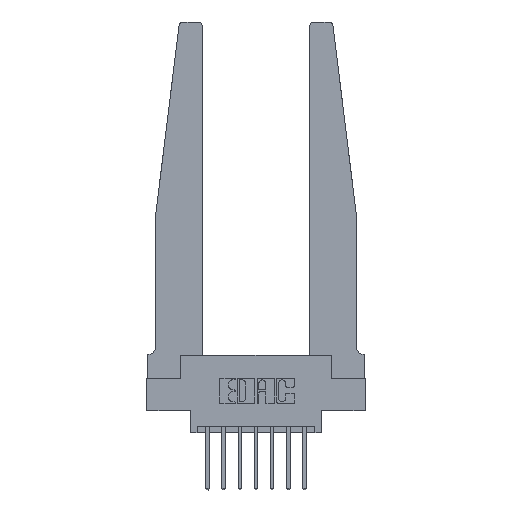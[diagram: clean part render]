
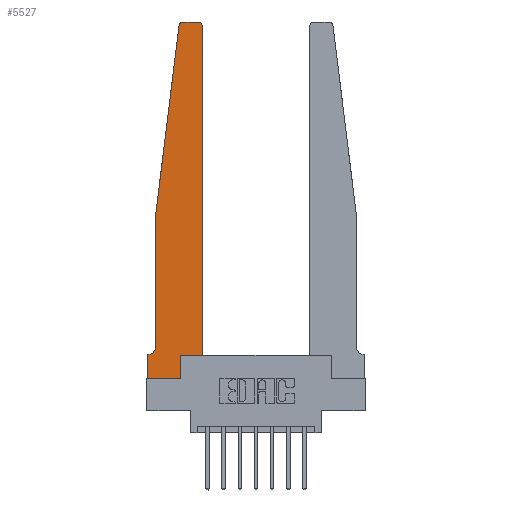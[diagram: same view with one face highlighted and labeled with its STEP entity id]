
A CAD part, top view. The second image highlights one B-rep face of the part: STEP entity #5527.
In plain terms, the highlighted planar face has unit normal (0, 0, 1).
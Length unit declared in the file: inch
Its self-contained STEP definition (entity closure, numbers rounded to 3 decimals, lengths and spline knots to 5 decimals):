
#216 = DIRECTION ( 'NONE',  ( 1., 0., 0. ) ) ;
#310 = LINE ( 'NONE', #7128, #11716 ) ;
#363 = CARTESIAN_POINT ( 'NONE',  ( 0., 0.1875, 0.37 ) ) ;
#381 = VERTEX_POINT ( 'NONE', #6612 ) ;
#487 = DIRECTION ( 'NONE',  ( 1., 0., 0. ) ) ;
#540 = AXIS2_PLACEMENT_3D ( 'NONE', #3076, #10787, #4205 ) ;
#876 = EDGE_CURVE ( 'NONE', #5665, #3880, #6739, .T. ) ;
#1044 = CARTESIAN_POINT ( 'NONE',  ( 0.065, 0.2375, 0.37 ) ) ;
#1462 = DIRECTION ( 'NONE',  ( 1., 0., 0. ) ) ;
#1758 = VERTEX_POINT ( 'NONE', #11754 ) ;
#2474 = CARTESIAN_POINT ( 'NONE',  ( 0.27653, 2.75, 0.37 ) ) ;
#2569 = EDGE_CURVE ( 'NONE', #6845, #3914, #9771, .T. ) ;
#2749 = CARTESIAN_POINT ( 'NONE',  ( 0.065, 1.25, 0.37 ) ) ;
#2785 = AXIS2_PLACEMENT_3D ( 'NONE', #363, #8144, #1462 ) ;
#3076 = CARTESIAN_POINT ( 'NONE',  ( 0.015, 0.2375, 0.37 ) ) ;
#3339 = CARTESIAN_POINT ( 'NONE',  ( 0.395, 2.72, 0.37 ) ) ;
#3422 = VERTEX_POINT ( 'NONE', #7314 ) ;
#3880 = VERTEX_POINT ( 'NONE', #2474 ) ;
#3914 = VERTEX_POINT ( 'NONE', #5905 ) ;
#4049 = VECTOR ( 'NONE', #8165, 39.37008 ) ;
#4205 = DIRECTION ( 'NONE',  ( -1., 0., 0. ) ) ;
#4410 = LINE ( 'NONE', #7078, #4049 ) ;
#4476 = DIRECTION ( 'NONE',  ( 1., 0., 0. ) ) ;
#4564 = VERTEX_POINT ( 'NONE', #6049 ) ;
#4570 = EDGE_CURVE ( 'NONE', #8054, #1758, #8384, .T. ) ;
#4601 = DIRECTION ( 'NONE',  ( 0., -1., 0. ) ) ;
#4630 = EDGE_CURVE ( 'NONE', #4564, #3422, #13072, .T. ) ;
#4813 = LINE ( 'NONE', #9383, #10650 ) ;
#4872 = DIRECTION ( 'NONE',  ( 0., 1., 0. ) ) ;
#4926 = DIRECTION ( 'NONE',  ( 0., 1., 0. ) ) ;
#4988 = ORIENTED_EDGE ( 'NONE', *, *, #11833, .T. ) ;
#5035 = CARTESIAN_POINT ( 'NONE',  ( 0.24675, 2.72367, 0.37 ) ) ;
#5098 = LINE ( 'NONE', #10093, #13069 ) ;
#5179 = VERTEX_POINT ( 'NONE', #5274 ) ;
#5274 = CARTESIAN_POINT ( 'NONE',  ( 0., 0.1875, 0.37 ) ) ;
#5280 = ORIENTED_EDGE ( 'NONE', *, *, #876, .T. ) ;
#5296 = VERTEX_POINT ( 'NONE', #1044 ) ;
#5505 = ORIENTED_EDGE ( 'NONE', *, *, #2569, .T. ) ;
#5527 = ADVANCED_FACE ( 'NONE', ( #11909 ), #7052, .T. ) ;
#5572 = ORIENTED_EDGE ( 'NONE', *, *, #10701, .T. ) ;
#5577 = CIRCLE ( 'NONE', #13024, 0.03 ) ;
#5595 = AXIS2_PLACEMENT_3D ( 'NONE', #3339, #11044, #4476 ) ;
#5665 = VERTEX_POINT ( 'NONE', #8442 ) ;
#5833 = CARTESIAN_POINT ( 'NONE',  ( 0.015, 0.1875, 0.37 ) ) ;
#5837 = ORIENTED_EDGE ( 'NONE', *, *, #13980, .T. ) ;
#5847 = ORIENTED_EDGE ( 'NONE', *, *, #13788, .T. ) ;
#5905 = CARTESIAN_POINT ( 'NONE',  ( 0.065, 1.25, 0.37 ) ) ;
#5926 = ORIENTED_EDGE ( 'NONE', *, *, #4570, .T. ) ;
#5956 = ORIENTED_EDGE ( 'NONE', *, *, #9748, .T. ) ;
#5977 = ORIENTED_EDGE ( 'NONE', *, *, #4630, .T. ) ;
#5992 = ORIENTED_EDGE ( 'NONE', *, *, #6795, .T. ) ;
#6049 = CARTESIAN_POINT ( 'NONE',  ( 0.2605, 0.18, 0.37 ) ) ;
#6101 = ORIENTED_EDGE ( 'NONE', *, *, #13414, .T. ) ;
#6612 = CARTESIAN_POINT ( 'NONE',  ( 0.425, 2.72, 0.37 ) ) ;
#6739 = LINE ( 'NONE', #6934, #12163 ) ;
#6772 = EDGE_CURVE ( 'NONE', #1758, #4564, #310, .T. ) ;
#6795 = EDGE_CURVE ( 'NONE', #3422, #381, #11359, .T. ) ;
#6845 = VERTEX_POINT ( 'NONE', #5035 ) ;
#6913 = DIRECTION ( 'NONE',  ( 0., 0., 1. ) ) ;
#6934 = CARTESIAN_POINT ( 'NONE',  ( 0.25, 2.75, 0.37 ) ) ;
#7052 = PLANE ( 'NONE',  #2785 ) ;
#7078 = CARTESIAN_POINT ( 'NONE',  ( 0., 0., 0.37 ) ) ;
#7128 = CARTESIAN_POINT ( 'NONE',  ( 0.2605, 0.18, 0.37 ) ) ;
#7208 = DIRECTION ( 'NONE',  ( -1., 0., 0. ) ) ;
#7219 = VERTEX_POINT ( 'NONE', #5833 ) ;
#7314 = CARTESIAN_POINT ( 'NONE',  ( 0.425, 0.18, 0.37 ) ) ;
#7382 = CARTESIAN_POINT ( 'NONE',  ( 0.425, 0.18, 0.37 ) ) ;
#8048 = VECTOR ( 'NONE', #487, 39.37008 ) ;
#8054 = VERTEX_POINT ( 'NONE', #9561 ) ;
#8144 = DIRECTION ( 'NONE',  ( 0., 0., 1. ) ) ;
#8165 = DIRECTION ( 'NONE',  ( 0., -1., 0. ) ) ;
#8384 = LINE ( 'NONE', #12549, #8048 ) ;
#8442 = CARTESIAN_POINT ( 'NONE',  ( 0.395, 2.75, 0.37 ) ) ;
#8470 = DIRECTION ( 'NONE',  ( 1., 0., 0. ) ) ;
#8634 = CIRCLE ( 'NONE', #540, 0.05 ) ;
#9040 = ORIENTED_EDGE ( 'NONE', *, *, #6772, .T. ) ;
#9383 = CARTESIAN_POINT ( 'NONE',  ( 0.065, 0.1875, 0.37 ) ) ;
#9561 = CARTESIAN_POINT ( 'NONE',  ( 0., 0., 0.37 ) ) ;
#9748 = EDGE_CURVE ( 'NONE', #5179, #8054, #4410, .T. ) ;
#9771 = LINE ( 'NONE', #2749, #12619 ) ;
#10093 = CARTESIAN_POINT ( 'NONE',  ( 0.065, 1.25, 0.37 ) ) ;
#10209 = DIRECTION ( 'NONE',  ( -1., 0., 0. ) ) ;
#10233 = VECTOR ( 'NONE', #8470, 39.37008 ) ;
#10650 = VECTOR ( 'NONE', #7208, 39.37008 ) ;
#10701 = EDGE_CURVE ( 'NONE', #3914, #5296, #5098, .T. ) ;
#10787 = DIRECTION ( 'NONE',  ( 0., 0., -1. ) ) ;
#11044 = DIRECTION ( 'NONE',  ( 0., 0., 1. ) ) ;
#11316 = EDGE_LOOP ( 'NONE', ( #5280, #4988, #5505, #5572, #5837, #5847, #5956, #5926, #9040, #5977, #5992, #6101 ) ) ;
#11359 = LINE ( 'NONE', #12546, #14203 ) ;
#11389 = DIRECTION ( 'NONE',  ( -0.122, -0.992, 0. ) ) ;
#11716 = VECTOR ( 'NONE', #4872, 39.37008 ) ;
#11754 = CARTESIAN_POINT ( 'NONE',  ( 0.2605, 0., 0.37 ) ) ;
#11833 = EDGE_CURVE ( 'NONE', #3880, #6845, #5577, .T. ) ;
#11862 = CIRCLE ( 'NONE', #5595, 0.03 ) ;
#11909 = FACE_OUTER_BOUND ( 'NONE', #11316, .T. ) ;
#12163 = VECTOR ( 'NONE', #10209, 39.37008 ) ;
#12546 = CARTESIAN_POINT ( 'NONE',  ( 0.425, 0.18, 0.37 ) ) ;
#12549 = CARTESIAN_POINT ( 'NONE',  ( 0., 0., 0.37 ) ) ;
#12619 = VECTOR ( 'NONE', #11389, 39.37008 ) ;
#13024 = AXIS2_PLACEMENT_3D ( 'NONE', #13346, #6913, #216 ) ;
#13069 = VECTOR ( 'NONE', #4601, 39.37008 ) ;
#13072 = LINE ( 'NONE', #7382, #10233 ) ;
#13346 = CARTESIAN_POINT ( 'NONE',  ( 0.27653, 2.72, 0.37 ) ) ;
#13414 = EDGE_CURVE ( 'NONE', #381, #5665, #11862, .T. ) ;
#13788 = EDGE_CURVE ( 'NONE', #7219, #5179, #4813, .T. ) ;
#13980 = EDGE_CURVE ( 'NONE', #5296, #7219, #8634, .T. ) ;
#14203 = VECTOR ( 'NONE', #4926, 39.37008 ) ;
